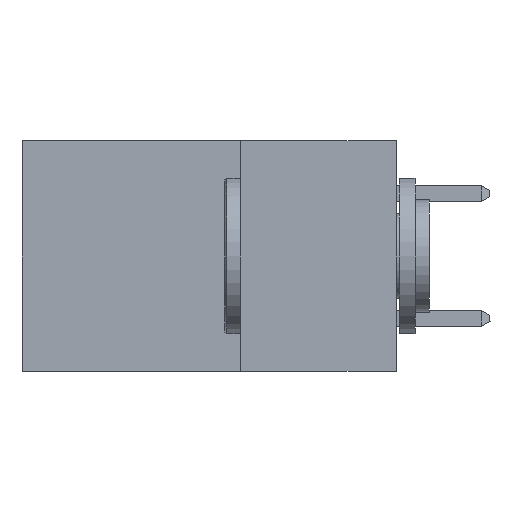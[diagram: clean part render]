
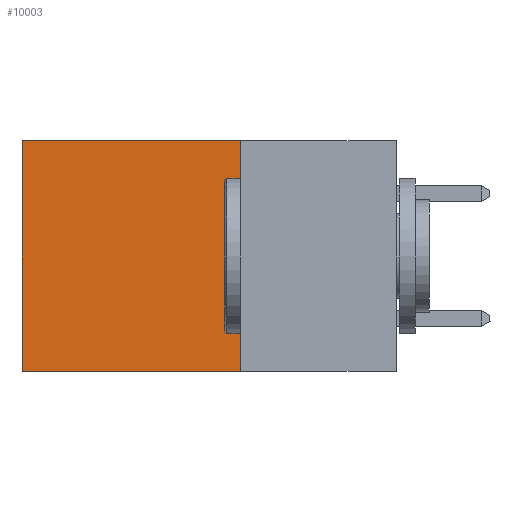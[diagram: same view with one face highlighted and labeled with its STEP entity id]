
A CAD part, left-side view. The second image highlights one B-rep face of the part: STEP entity #10003.
In plain terms, the highlighted planar face has unit normal (-1, 0, 0).
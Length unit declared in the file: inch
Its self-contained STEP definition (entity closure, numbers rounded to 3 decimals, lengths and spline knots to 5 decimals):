
#1433 = ORIENTED_EDGE ( 'NONE', *, *, #20903, .F. ) ;
#1959 = VERTEX_POINT ( 'NONE', #8378 ) ;
#1987 = VERTEX_POINT ( 'NONE', #7971 ) ;
#2637 = LINE ( 'NONE', #7800, #22855 ) ;
#3711 = CARTESIAN_POINT ( 'NONE',  ( 0.2615, 0.25, -0.37 ) ) ;
#5410 = VECTOR ( 'NONE', #22953, 39.37008 ) ;
#5549 = EDGE_CURVE ( 'NONE', #1987, #15152, #15579, .T. ) ;
#6022 = CARTESIAN_POINT ( 'NONE',  ( 0.2615, 0.25, 0. ) ) ;
#6063 = ORIENTED_EDGE ( 'NONE', *, *, #10825, .T. ) ;
#6084 = CARTESIAN_POINT ( 'NONE',  ( 0.2615, 0.6, -0.37 ) ) ;
#7005 = CARTESIAN_POINT ( 'NONE',  ( 0.2615, 0.25, -0.37 ) ) ;
#7109 = EDGE_CURVE ( 'NONE', #1959, #15152, #2637, .T. ) ;
#7573 = DIRECTION ( 'NONE',  ( 0., 0., -1. ) ) ;
#7800 = CARTESIAN_POINT ( 'NONE',  ( 0.2615, 0.6, -0.37 ) ) ;
#7867 = CARTESIAN_POINT ( 'NONE',  ( 0.2615, 0.25, 0. ) ) ;
#7971 = CARTESIAN_POINT ( 'NONE',  ( 0.2615, 0.25, -0.37 ) ) ;
#8231 = LINE ( 'NONE', #7005, #22145 ) ;
#8378 = CARTESIAN_POINT ( 'NONE',  ( 0.2615, 0.6, 0. ) ) ;
#9411 = VERTEX_POINT ( 'NONE', #6022 ) ;
#10003 = ADVANCED_FACE ( 'NONE', ( #17606 ), #17063, .F. ) ;
#10825 = EDGE_CURVE ( 'NONE', #9411, #1959, #18750, .T. ) ;
#11436 = EDGE_LOOP ( 'NONE', ( #20513, #22463, #1433, #6063 ) ) ;
#13727 = VECTOR ( 'NONE', #21136, 39.37008 ) ;
#15152 = VERTEX_POINT ( 'NONE', #6084 ) ;
#15579 = LINE ( 'NONE', #23909, #5410 ) ;
#17063 = PLANE ( 'NONE',  #18506 ) ;
#17606 = FACE_OUTER_BOUND ( 'NONE', #11436, .T. ) ;
#18407 = DIRECTION ( 'NONE',  ( 0., 0., -1. ) ) ;
#18506 = AXIS2_PLACEMENT_3D ( 'NONE', #3711, #18978, #7573 ) ;
#18750 = LINE ( 'NONE', #7867, #13727 ) ;
#18978 = DIRECTION ( 'NONE',  ( 1., 0., 0. ) ) ;
#20513 = ORIENTED_EDGE ( 'NONE', *, *, #7109, .T. ) ;
#20903 = EDGE_CURVE ( 'NONE', #9411, #1987, #8231, .T. ) ;
#21065 = DIRECTION ( 'NONE',  ( 0., 0., -1. ) ) ;
#21136 = DIRECTION ( 'NONE',  ( 0., 1., 0. ) ) ;
#22145 = VECTOR ( 'NONE', #18407, 39.37008 ) ;
#22463 = ORIENTED_EDGE ( 'NONE', *, *, #5549, .F. ) ;
#22855 = VECTOR ( 'NONE', #21065, 39.37008 ) ;
#22953 = DIRECTION ( 'NONE',  ( 0., 1., 0. ) ) ;
#23909 = CARTESIAN_POINT ( 'NONE',  ( 0.2615, 0.25, -0.37 ) ) ;
